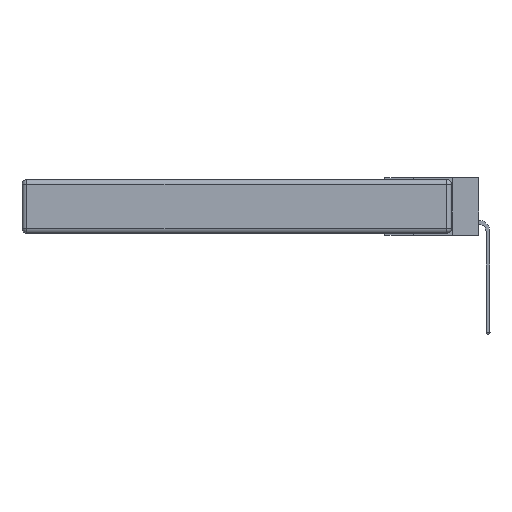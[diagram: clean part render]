
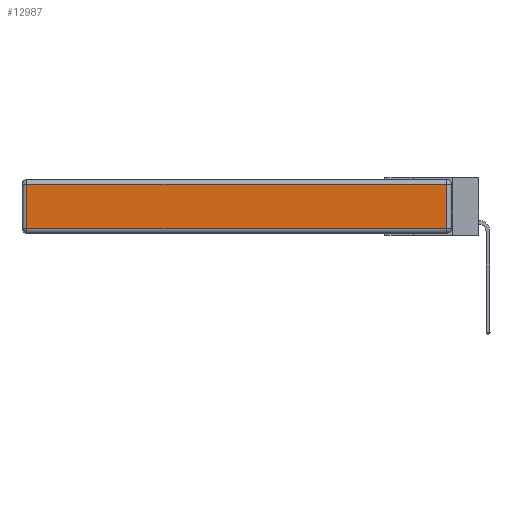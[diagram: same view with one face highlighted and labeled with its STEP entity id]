
A CAD part, left-side view. The second image highlights one B-rep face of the part: STEP entity #12987.
In plain terms, the highlighted planar face has unit normal (-1, 0, 0).
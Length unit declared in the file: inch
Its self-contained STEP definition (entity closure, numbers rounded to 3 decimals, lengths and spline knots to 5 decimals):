
#213 = LINE ( 'NONE', #4896, #11159 ) ;
#1680 = VECTOR ( 'NONE', #5220, 39.37008 ) ;
#1712 = CARTESIAN_POINT ( 'NONE',  ( 0., 0.03, -0.313 ) ) ;
#2002 = ORIENTED_EDGE ( 'NONE', *, *, #9721, .T. ) ;
#2790 = DIRECTION ( 'NONE',  ( 0., 0., -1. ) ) ;
#2941 = CARTESIAN_POINT ( 'NONE',  ( 0., 2.72, -0.03 ) ) ;
#3159 = LINE ( 'NONE', #8228, #1680 ) ;
#3535 = CARTESIAN_POINT ( 'NONE',  ( 0., 0., -0.313 ) ) ;
#4003 = CARTESIAN_POINT ( 'NONE',  ( 0., 0.03, -0.03 ) ) ;
#4454 = PLANE ( 'NONE',  #4471 ) ;
#4471 = AXIS2_PLACEMENT_3D ( 'NONE', #6716, #11903, #12095 ) ;
#4576 = DIRECTION ( 'NONE',  ( 0., -1., 0. ) ) ;
#4896 = CARTESIAN_POINT ( 'NONE',  ( 0., 2.75, -0.03 ) ) ;
#5220 = DIRECTION ( 'NONE',  ( 0., 0., 1. ) ) ;
#5635 = VERTEX_POINT ( 'NONE', #1712 ) ;
#6336 = EDGE_CURVE ( 'NONE', #10014, #5635, #12524, .T. ) ;
#6716 = CARTESIAN_POINT ( 'NONE',  ( 0., 0., -0.343 ) ) ;
#7003 = EDGE_CURVE ( 'NONE', #7718, #12983, #213, .T. ) ;
#7437 = LINE ( 'NONE', #8110, #12802 ) ;
#7718 = VERTEX_POINT ( 'NONE', #4003 ) ;
#8110 = CARTESIAN_POINT ( 'NONE',  ( 0., 2.72, -0.343 ) ) ;
#8228 = CARTESIAN_POINT ( 'NONE',  ( 0., 0.03, -0.343 ) ) ;
#8344 = ORIENTED_EDGE ( 'NONE', *, *, #7003, .T. ) ;
#8752 = FACE_OUTER_BOUND ( 'NONE', #12110, .T. ) ;
#9666 = VECTOR ( 'NONE', #4576, 39.37008 ) ;
#9721 = EDGE_CURVE ( 'NONE', #5635, #7718, #3159, .T. ) ;
#10014 = VERTEX_POINT ( 'NONE', #13245 ) ;
#10654 = ORIENTED_EDGE ( 'NONE', *, *, #11393, .T. ) ;
#10978 = ORIENTED_EDGE ( 'NONE', *, *, #6336, .T. ) ;
#11159 = VECTOR ( 'NONE', #12399, 39.37008 ) ;
#11393 = EDGE_CURVE ( 'NONE', #12983, #10014, #7437, .T. ) ;
#11903 = DIRECTION ( 'NONE',  ( -1., 0., 0. ) ) ;
#12095 = DIRECTION ( 'NONE',  ( 0., 0., 1. ) ) ;
#12110 = EDGE_LOOP ( 'NONE', ( #10978, #2002, #8344, #10654 ) ) ;
#12399 = DIRECTION ( 'NONE',  ( 0., 1., 0. ) ) ;
#12524 = LINE ( 'NONE', #3535, #9666 ) ;
#12802 = VECTOR ( 'NONE', #2790, 39.37008 ) ;
#12983 = VERTEX_POINT ( 'NONE', #2941 ) ;
#12987 = ADVANCED_FACE ( 'NONE', ( #8752 ), #4454, .T. ) ;
#13245 = CARTESIAN_POINT ( 'NONE',  ( 0., 2.72, -0.313 ) ) ;
